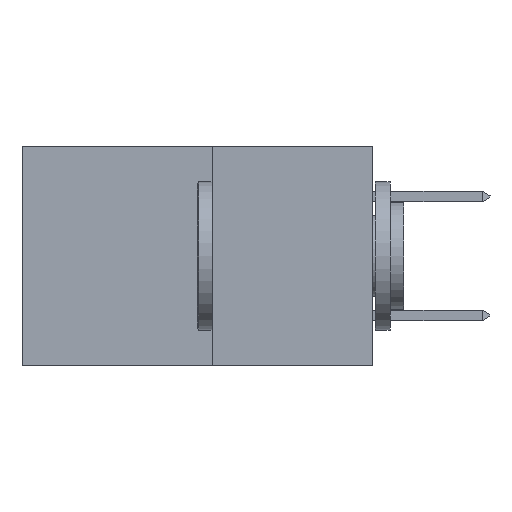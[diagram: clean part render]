
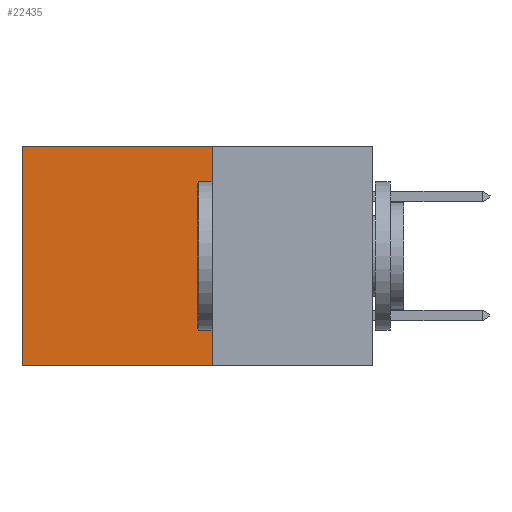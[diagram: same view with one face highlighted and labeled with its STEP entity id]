
A CAD part, left-side view. The second image highlights one B-rep face of the part: STEP entity #22435.
In plain terms, the highlighted planar face has unit normal (-1, 0, 0).
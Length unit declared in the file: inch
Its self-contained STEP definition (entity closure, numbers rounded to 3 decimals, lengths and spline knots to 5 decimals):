
#9 = VERTEX_POINT ( 'NONE', #30726 ) ;
#3240 = CARTESIAN_POINT ( 'NONE',  ( 0.277, 0.27, 0. ) ) ;
#3478 = ORIENTED_EDGE ( 'NONE', *, *, #17626, .T. ) ;
#3885 = DIRECTION ( 'NONE',  ( 0., 0., -1. ) ) ;
#3944 = VECTOR ( 'NONE', #15351, 39.37008 ) ;
#4796 = VERTEX_POINT ( 'NONE', #20876 ) ;
#6221 = CARTESIAN_POINT ( 'NONE',  ( 0.277, 0.27, -0.37 ) ) ;
#6867 = PLANE ( 'NONE',  #10316 ) ;
#7220 = EDGE_CURVE ( 'NONE', #9, #16042, #12301, .T. ) ;
#8141 = DIRECTION ( 'NONE',  ( 0., 1., 0. ) ) ;
#9030 = EDGE_LOOP ( 'NONE', ( #3478, #21855, #11535, #16598 ) ) ;
#9359 = DIRECTION ( 'NONE',  ( 1., 0., 0. ) ) ;
#10316 = AXIS2_PLACEMENT_3D ( 'NONE', #23833, #9359, #26247 ) ;
#10470 = LINE ( 'NONE', #12904, #3944 ) ;
#11535 = ORIENTED_EDGE ( 'NONE', *, *, #13407, .F. ) ;
#12301 = LINE ( 'NONE', #19040, #24356 ) ;
#12904 = CARTESIAN_POINT ( 'NONE',  ( 0.277, 0.59, -0.37 ) ) ;
#13037 = VECTOR ( 'NONE', #8141, 39.37008 ) ;
#13407 = EDGE_CURVE ( 'NONE', #17763, #9, #17584, .T. ) ;
#15351 = DIRECTION ( 'NONE',  ( 0., 0., -1. ) ) ;
#16042 = VERTEX_POINT ( 'NONE', #30798 ) ;
#16598 = ORIENTED_EDGE ( 'NONE', *, *, #19835, .T. ) ;
#17584 = LINE ( 'NONE', #6221, #28817 ) ;
#17626 = EDGE_CURVE ( 'NONE', #4796, #16042, #10470, .T. ) ;
#17763 = VERTEX_POINT ( 'NONE', #25400 ) ;
#18687 = LINE ( 'NONE', #3240, #13037 ) ;
#18906 = DIRECTION ( 'NONE',  ( 0., 1., 0. ) ) ;
#19040 = CARTESIAN_POINT ( 'NONE',  ( 0.277, 0.27, -0.37 ) ) ;
#19835 = EDGE_CURVE ( 'NONE', #17763, #4796, #18687, .T. ) ;
#20876 = CARTESIAN_POINT ( 'NONE',  ( 0.277, 0.59, 0. ) ) ;
#21855 = ORIENTED_EDGE ( 'NONE', *, *, #7220, .F. ) ;
#22435 = ADVANCED_FACE ( 'NONE', ( #23835 ), #6867, .F. ) ;
#23833 = CARTESIAN_POINT ( 'NONE',  ( 0.277, 0.27, -0.37 ) ) ;
#23835 = FACE_OUTER_BOUND ( 'NONE', #9030, .T. ) ;
#24356 = VECTOR ( 'NONE', #18906, 39.37008 ) ;
#25400 = CARTESIAN_POINT ( 'NONE',  ( 0.277, 0.27, 0. ) ) ;
#26247 = DIRECTION ( 'NONE',  ( 0., 0., -1. ) ) ;
#28817 = VECTOR ( 'NONE', #3885, 39.37008 ) ;
#30726 = CARTESIAN_POINT ( 'NONE',  ( 0.277, 0.27, -0.37 ) ) ;
#30798 = CARTESIAN_POINT ( 'NONE',  ( 0.277, 0.59, -0.37 ) ) ;
